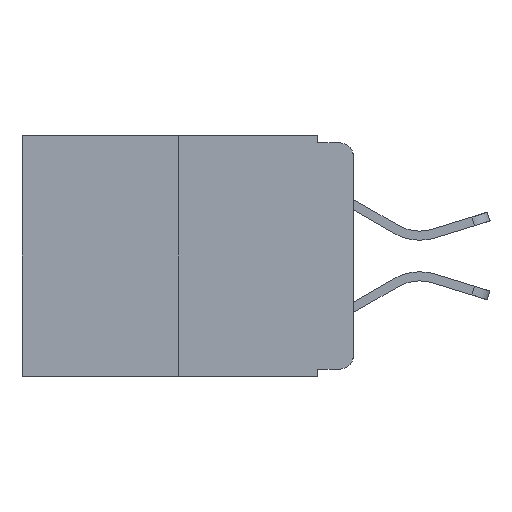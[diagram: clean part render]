
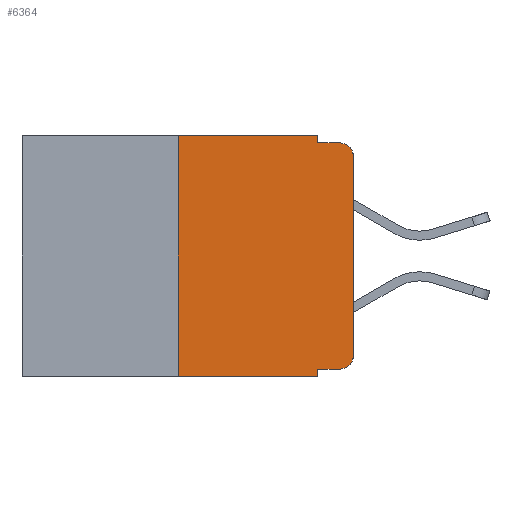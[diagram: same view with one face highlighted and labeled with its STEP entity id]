
A CAD part, left-side view. The second image highlights one B-rep face of the part: STEP entity #6364.
In plain terms, the highlighted planar face has unit normal (-1, 0, 0).
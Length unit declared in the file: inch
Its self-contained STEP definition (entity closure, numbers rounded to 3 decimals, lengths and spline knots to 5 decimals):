
#31 = EDGE_CURVE ( 'NONE', #5026, #11219, #1329, .T. ) ;
#57 = ORIENTED_EDGE ( 'NONE', *, *, #1524, .T. ) ;
#60 = LINE ( 'NONE', #2695, #9685 ) ;
#644 = EDGE_LOOP ( 'NONE', ( #672, #810, #934, #2042, #3246, #6261, #6618, #4670, #7945, #57 ) ) ;
#672 = ORIENTED_EDGE ( 'NONE', *, *, #8512, .T. ) ;
#709 = VECTOR ( 'NONE', #10792, 39.37008 ) ;
#764 = DIRECTION ( 'NONE',  ( 0., 0., -1. ) ) ;
#787 = EDGE_CURVE ( 'NONE', #5026, #4047, #60, .T. ) ;
#810 = ORIENTED_EDGE ( 'NONE', *, *, #9066, .T. ) ;
#819 = VERTEX_POINT ( 'NONE', #2652 ) ;
#934 = ORIENTED_EDGE ( 'NONE', *, *, #9634, .F. ) ;
#979 = VECTOR ( 'NONE', #6063, 39.37008 ) ;
#981 = VERTEX_POINT ( 'NONE', #3634 ) ;
#1329 = LINE ( 'NONE', #2544, #979 ) ;
#1423 = DIRECTION ( 'NONE',  ( 0., -1., 0. ) ) ;
#1524 = EDGE_CURVE ( 'NONE', #4047, #819, #8179, .T. ) ;
#1586 = VERTEX_POINT ( 'NONE', #6685 ) ;
#1778 = DIRECTION ( 'NONE',  ( 0., -1., 0. ) ) ;
#1780 = CIRCLE ( 'NONE', #11032, 0.02 ) ;
#2042 = ORIENTED_EDGE ( 'NONE', *, *, #10221, .F. ) ;
#2132 = VERTEX_POINT ( 'NONE', #6600 ) ;
#2371 = AXIS2_PLACEMENT_3D ( 'NONE', #9617, #2479, #11138 ) ;
#2453 = VERTEX_POINT ( 'NONE', #3494 ) ;
#2479 = DIRECTION ( 'NONE',  ( 1., 0., 0. ) ) ;
#2528 = DIRECTION ( 'NONE',  ( 0., -1., 0. ) ) ;
#2544 = CARTESIAN_POINT ( 'NONE',  ( 0., 0.051, 0. ) ) ;
#2652 = CARTESIAN_POINT ( 'NONE',  ( 0., 0., -0.313 ) ) ;
#2695 = CARTESIAN_POINT ( 'NONE',  ( 0., 0.051, -0.333 ) ) ;
#2780 = VERTEX_POINT ( 'NONE', #3189 ) ;
#3189 = CARTESIAN_POINT ( 'NONE',  ( 0., 0.051, -0.01 ) ) ;
#3246 = ORIENTED_EDGE ( 'NONE', *, *, #11623, .F. ) ;
#3438 = DIRECTION ( 'NONE',  ( 0., 0., -1. ) ) ;
#3494 = CARTESIAN_POINT ( 'NONE',  ( 0., 0.25, -0.343 ) ) ;
#3538 = DIRECTION ( 'NONE',  ( 0., 0., 1. ) ) ;
#3634 = CARTESIAN_POINT ( 'NONE',  ( 0., 0., -0.03 ) ) ;
#4047 = VERTEX_POINT ( 'NONE', #11536 ) ;
#4080 = DIRECTION ( 'NONE',  ( 0., -1., 0. ) ) ;
#4656 = CARTESIAN_POINT ( 'NONE',  ( 0., 0., 0. ) ) ;
#4670 = ORIENTED_EDGE ( 'NONE', *, *, #31, .F. ) ;
#4960 = VECTOR ( 'NONE', #2528, 39.37008 ) ;
#4981 = CARTESIAN_POINT ( 'NONE',  ( 0., 0.473, 0. ) ) ;
#5026 = VERTEX_POINT ( 'NONE', #10114 ) ;
#5231 = VECTOR ( 'NONE', #1423, 39.37008 ) ;
#5415 = AXIS2_PLACEMENT_3D ( 'NONE', #9033, #11486, #11422 ) ;
#5760 = LINE ( 'NONE', #4656, #709 ) ;
#6063 = DIRECTION ( 'NONE',  ( 0., 0., -1. ) ) ;
#6091 = CARTESIAN_POINT ( 'NONE',  ( 0., 0.051, 0. ) ) ;
#6182 = CARTESIAN_POINT ( 'NONE',  ( 0., 0.051, 0. ) ) ;
#6261 = ORIENTED_EDGE ( 'NONE', *, *, #10766, .F. ) ;
#6358 = FACE_OUTER_BOUND ( 'NONE', #644, .T. ) ;
#6364 = ADVANCED_FACE ( 'NONE', ( #6358 ), #10267, .F. ) ;
#6393 = DIRECTION ( 'NONE',  ( -1., 0., 0. ) ) ;
#6565 = VECTOR ( 'NONE', #4080, 39.37008 ) ;
#6600 = CARTESIAN_POINT ( 'NONE',  ( 0., 0.02, -0.01 ) ) ;
#6618 = ORIENTED_EDGE ( 'NONE', *, *, #9578, .T. ) ;
#6685 = CARTESIAN_POINT ( 'NONE',  ( 0., 0.25, 0. ) ) ;
#7072 = CARTESIAN_POINT ( 'NONE',  ( 0., 0.051, -0.343 ) ) ;
#7144 = LINE ( 'NONE', #4981, #6565 ) ;
#7619 = LINE ( 'NONE', #8746, #5231 ) ;
#7945 = ORIENTED_EDGE ( 'NONE', *, *, #787, .T. ) ;
#8179 = CIRCLE ( 'NONE', #5415, 0.02 ) ;
#8319 = VECTOR ( 'NONE', #3438, 39.37008 ) ;
#8330 = VERTEX_POINT ( 'NONE', #6182 ) ;
#8512 = EDGE_CURVE ( 'NONE', #819, #981, #5760, .T. ) ;
#8746 = CARTESIAN_POINT ( 'NONE',  ( 0., 0.473, -0.343 ) ) ;
#9033 = CARTESIAN_POINT ( 'NONE',  ( 0., 0.02, -0.313 ) ) ;
#9066 = EDGE_CURVE ( 'NONE', #981, #2132, #1780, .T. ) ;
#9243 = LINE ( 'NONE', #11369, #10941 ) ;
#9578 = EDGE_CURVE ( 'NONE', #2453, #11219, #7619, .T. ) ;
#9617 = CARTESIAN_POINT ( 'NONE',  ( 0., 0.473, 0. ) ) ;
#9634 = EDGE_CURVE ( 'NONE', #2780, #2132, #9670, .T. ) ;
#9658 = CARTESIAN_POINT ( 'NONE',  ( 0., 0.051, -0.01 ) ) ;
#9670 = LINE ( 'NONE', #9658, #4960 ) ;
#9685 = VECTOR ( 'NONE', #1778, 39.37008 ) ;
#10114 = CARTESIAN_POINT ( 'NONE',  ( 0., 0.051, -0.333 ) ) ;
#10221 = EDGE_CURVE ( 'NONE', #8330, #2780, #10579, .T. ) ;
#10267 = PLANE ( 'NONE',  #2371 ) ;
#10579 = LINE ( 'NONE', #6091, #8319 ) ;
#10766 = EDGE_CURVE ( 'NONE', #2453, #1586, #9243, .T. ) ;
#10792 = DIRECTION ( 'NONE',  ( 0., 0., 1. ) ) ;
#10941 = VECTOR ( 'NONE', #3538, 39.37008 ) ;
#11032 = AXIS2_PLACEMENT_3D ( 'NONE', #11526, #6393, #764 ) ;
#11138 = DIRECTION ( 'NONE',  ( 0., 0., -1. ) ) ;
#11219 = VERTEX_POINT ( 'NONE', #7072 ) ;
#11369 = CARTESIAN_POINT ( 'NONE',  ( 0., 0.25, 0. ) ) ;
#11422 = DIRECTION ( 'NONE',  ( 0., 0., -1. ) ) ;
#11486 = DIRECTION ( 'NONE',  ( -1., 0., 0. ) ) ;
#11526 = CARTESIAN_POINT ( 'NONE',  ( 0., 0.02, -0.03 ) ) ;
#11536 = CARTESIAN_POINT ( 'NONE',  ( 0., 0.02, -0.333 ) ) ;
#11623 = EDGE_CURVE ( 'NONE', #1586, #8330, #7144, .T. ) ;
